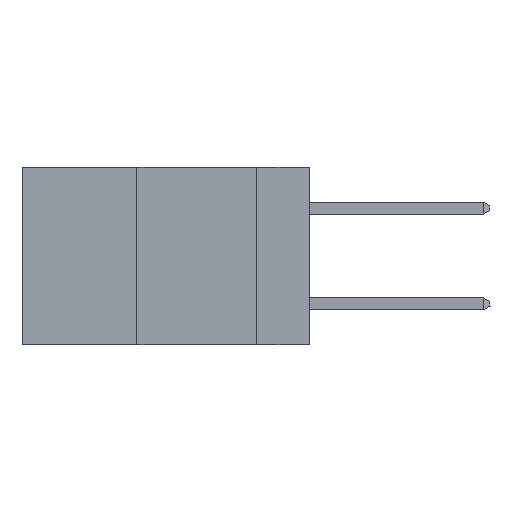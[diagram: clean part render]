
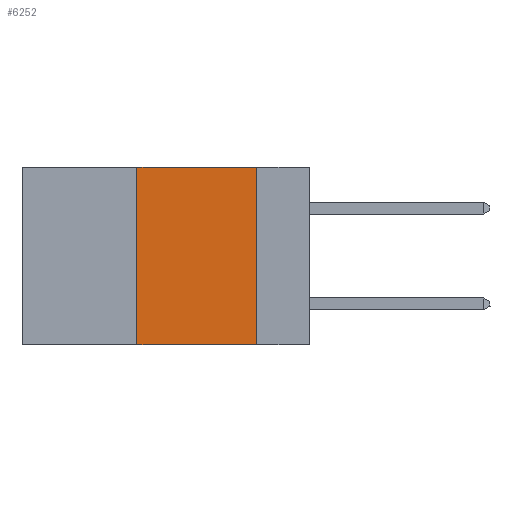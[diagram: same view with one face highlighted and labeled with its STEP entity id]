
A CAD part, left-side view. The second image highlights one B-rep face of the part: STEP entity #6252.
In plain terms, the highlighted planar face has unit normal (-1, 0, 0).
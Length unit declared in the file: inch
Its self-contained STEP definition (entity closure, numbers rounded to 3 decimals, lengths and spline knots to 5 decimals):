
#68 = DIRECTION ( 'NONE',  ( 0., -1., 0. ) ) ;
#132 = CARTESIAN_POINT ( 'NONE',  ( 0., 0.6, -0.37 ) ) ;
#667 = VERTEX_POINT ( 'NONE', #11403 ) ;
#957 = AXIS2_PLACEMENT_3D ( 'NONE', #6016, #9598, #21695 ) ;
#2781 = CARTESIAN_POINT ( 'NONE',  ( 0., 0.6, 0. ) ) ;
#3091 = FACE_OUTER_BOUND ( 'NONE', #18501, .T. ) ;
#3172 = VECTOR ( 'NONE', #8019, 39.37008 ) ;
#3970 = VECTOR ( 'NONE', #9945, 39.37008 ) ;
#4608 = CARTESIAN_POINT ( 'NONE',  ( 0., 0.11, 0. ) ) ;
#5090 = EDGE_CURVE ( 'NONE', #5337, #6769, #8687, .T. ) ;
#5337 = VERTEX_POINT ( 'NONE', #17423 ) ;
#6016 = CARTESIAN_POINT ( 'NONE',  ( 0., 0.6, 0. ) ) ;
#6252 = ADVANCED_FACE ( 'NONE', ( #3091 ), #19971, .F. ) ;
#6769 = VERTEX_POINT ( 'NONE', #7698 ) ;
#7441 = VECTOR ( 'NONE', #68, 39.37008 ) ;
#7698 = CARTESIAN_POINT ( 'NONE',  ( 0., 0.11, -0.37 ) ) ;
#7723 = EDGE_CURVE ( 'NONE', #667, #6769, #16723, .T. ) ;
#8019 = DIRECTION ( 'NONE',  ( 0., -1., 0. ) ) ;
#8687 = LINE ( 'NONE', #4608, #3970 ) ;
#9598 = DIRECTION ( 'NONE',  ( 1., 0., 0. ) ) ;
#9670 = DIRECTION ( 'NONE',  ( 0., 0., 1. ) ) ;
#9945 = DIRECTION ( 'NONE',  ( 0., 0., -1. ) ) ;
#10160 = VECTOR ( 'NONE', #9670, 39.37008 ) ;
#11403 = CARTESIAN_POINT ( 'NONE',  ( 0., 0.36, -0.37 ) ) ;
#13427 = ORIENTED_EDGE ( 'NONE', *, *, #16355, .F. ) ;
#13572 = EDGE_CURVE ( 'NONE', #20440, #5337, #17140, .T. ) ;
#15608 = CARTESIAN_POINT ( 'NONE',  ( 0., 0.36, 0. ) ) ;
#16355 = EDGE_CURVE ( 'NONE', #667, #20440, #19362, .T. ) ;
#16723 = LINE ( 'NONE', #132, #7441 ) ;
#17140 = LINE ( 'NONE', #2781, #3172 ) ;
#17423 = CARTESIAN_POINT ( 'NONE',  ( 0., 0.11, 0. ) ) ;
#18501 = EDGE_LOOP ( 'NONE', ( #18571, #20876, #13427, #18524 ) ) ;
#18524 = ORIENTED_EDGE ( 'NONE', *, *, #7723, .T. ) ;
#18571 = ORIENTED_EDGE ( 'NONE', *, *, #5090, .F. ) ;
#19362 = LINE ( 'NONE', #21769, #10160 ) ;
#19971 = PLANE ( 'NONE',  #957 ) ;
#20440 = VERTEX_POINT ( 'NONE', #15608 ) ;
#20876 = ORIENTED_EDGE ( 'NONE', *, *, #13572, .F. ) ;
#21695 = DIRECTION ( 'NONE',  ( 0., 0., -1. ) ) ;
#21769 = CARTESIAN_POINT ( 'NONE',  ( 0., 0.36, 0. ) ) ;
